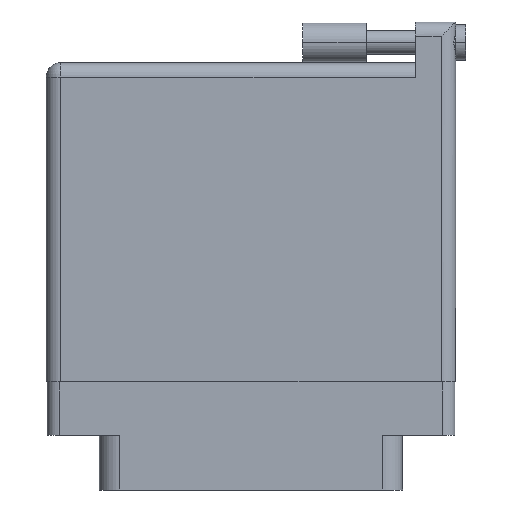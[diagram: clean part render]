
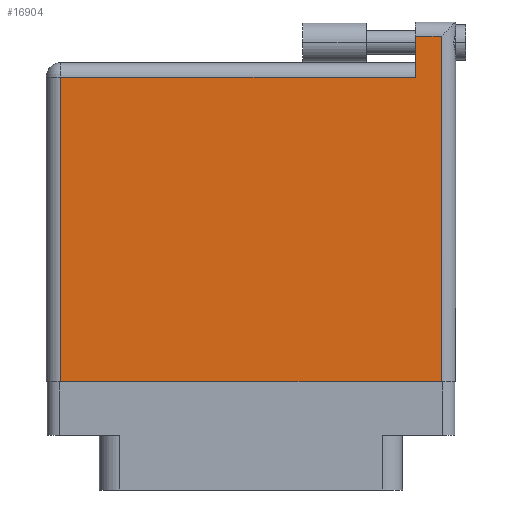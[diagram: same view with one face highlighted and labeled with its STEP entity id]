
A CAD part, front view. The second image highlights one B-rep face of the part: STEP entity #16904.
In plain terms, the highlighted face is planar.
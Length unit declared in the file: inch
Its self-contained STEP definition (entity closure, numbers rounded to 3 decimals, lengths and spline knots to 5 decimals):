
#1135 = EDGE_CURVE ( 'NONE', #28958, #35820, #31460, .T. ) ;
#3159 = CARTESIAN_POINT ( 'NONE',  ( 0., 1.496, 0. ) ) ;
#3808 = CARTESIAN_POINT ( 'NONE',  ( 1.811, 1.766, 0. ) ) ;
#3940 = DIRECTION ( 'NONE',  ( 0., -1., 0. ) ) ;
#4105 = VERTEX_POINT ( 'NONE', #19006 ) ;
#4518 = CARTESIAN_POINT ( 'NONE',  ( 0., 1.566, 0. ) ) ;
#4605 = VECTOR ( 'NONE', #8615, 39.37008 ) ;
#6702 = VERTEX_POINT ( 'NONE', #16336 ) ;
#6779 = DIRECTION ( 'NONE',  ( -1., 0., 0. ) ) ;
#7242 = VECTOR ( 'NONE', #13651, 39.37008 ) ;
#7459 = VERTEX_POINT ( 'NONE', #11804 ) ;
#7505 = ORIENTED_EDGE ( 'NONE', *, *, #16703, .T. ) ;
#8615 = DIRECTION ( 'NONE',  ( -1., 0., 0. ) ) ;
#10656 = CARTESIAN_POINT ( 'NONE',  ( 1.938, 1.766, 0. ) ) ;
#11670 = DIRECTION ( 'NONE',  ( 1., 0., 0. ) ) ;
#11804 = CARTESIAN_POINT ( 'NONE',  ( 0.07, 0., 0. ) ) ;
#13028 = DIRECTION ( 'NONE',  ( -1., 0., 0. ) ) ;
#13505 = CARTESIAN_POINT ( 'NONE',  ( 0.07, 0., 0. ) ) ;
#13651 = DIRECTION ( 'NONE',  ( 0., -1., 0. ) ) ;
#13669 = VECTOR ( 'NONE', #6779, 39.37008 ) ;
#14080 = ORIENTED_EDGE ( 'NONE', *, *, #1135, .T. ) ;
#14256 = AXIS2_PLACEMENT_3D ( 'NONE', #4518, #36982, #13028 ) ;
#14350 = VECTOR ( 'NONE', #11670, 39.37008 ) ;
#14381 = VECTOR ( 'NONE', #31510, 39.37008 ) ;
#15368 = LINE ( 'NONE', #3159, #4605 ) ;
#15834 = CARTESIAN_POINT ( 'NONE',  ( 0., 1.696, 0. ) ) ;
#16053 = PLANE ( 'NONE',  #14256 ) ;
#16336 = CARTESIAN_POINT ( 'NONE',  ( 1.938, 1.696, 0. ) ) ;
#16703 = EDGE_CURVE ( 'NONE', #35820, #4105, #15368, .T. ) ;
#16840 = ORIENTED_EDGE ( 'NONE', *, *, #36855, .T. ) ;
#16904 = ADVANCED_FACE ( 'NONE', ( #31773 ), #16053, .F. ) ;
#16925 = LINE ( 'NONE', #15834, #13669 ) ;
#18090 = CARTESIAN_POINT ( 'NONE',  ( 1.811, 1.696, 0. ) ) ;
#18674 = EDGE_CURVE ( 'NONE', #4105, #7459, #33029, .T. ) ;
#19006 = CARTESIAN_POINT ( 'NONE',  ( 0.07, 1.496, 0. ) ) ;
#24121 = CARTESIAN_POINT ( 'NONE',  ( 1.938, 0., 0. ) ) ;
#25624 = LINE ( 'NONE', #10656, #14381 ) ;
#26191 = EDGE_CURVE ( 'NONE', #6702, #28958, #16925, .T. ) ;
#27573 = CARTESIAN_POINT ( 'NONE',  ( 1.811, 1.496, 0. ) ) ;
#28469 = ORIENTED_EDGE ( 'NONE', *, *, #18674, .T. ) ;
#28958 = VERTEX_POINT ( 'NONE', #18090 ) ;
#30969 = VECTOR ( 'NONE', #3940, 39.37008 ) ;
#31460 = LINE ( 'NONE', #3808, #30969 ) ;
#31510 = DIRECTION ( 'NONE',  ( 0., 1., 0. ) ) ;
#31755 = ORIENTED_EDGE ( 'NONE', *, *, #26191, .T. ) ;
#31773 = FACE_OUTER_BOUND ( 'NONE', #32037, .T. ) ;
#31930 = VERTEX_POINT ( 'NONE', #24121 ) ;
#32037 = EDGE_LOOP ( 'NONE', ( #36120, #16840, #31755, #14080, #7505, #28469 ) ) ;
#33029 = LINE ( 'NONE', #13505, #7242 ) ;
#33555 = EDGE_CURVE ( 'NONE', #7459, #31930, #38236, .T. ) ;
#35202 = CARTESIAN_POINT ( 'NONE',  ( 0., 0., 0. ) ) ;
#35820 = VERTEX_POINT ( 'NONE', #27573 ) ;
#36120 = ORIENTED_EDGE ( 'NONE', *, *, #33555, .T. ) ;
#36855 = EDGE_CURVE ( 'NONE', #31930, #6702, #25624, .T. ) ;
#36982 = DIRECTION ( 'NONE',  ( 0., 0., -1. ) ) ;
#38236 = LINE ( 'NONE', #35202, #14350 ) ;
